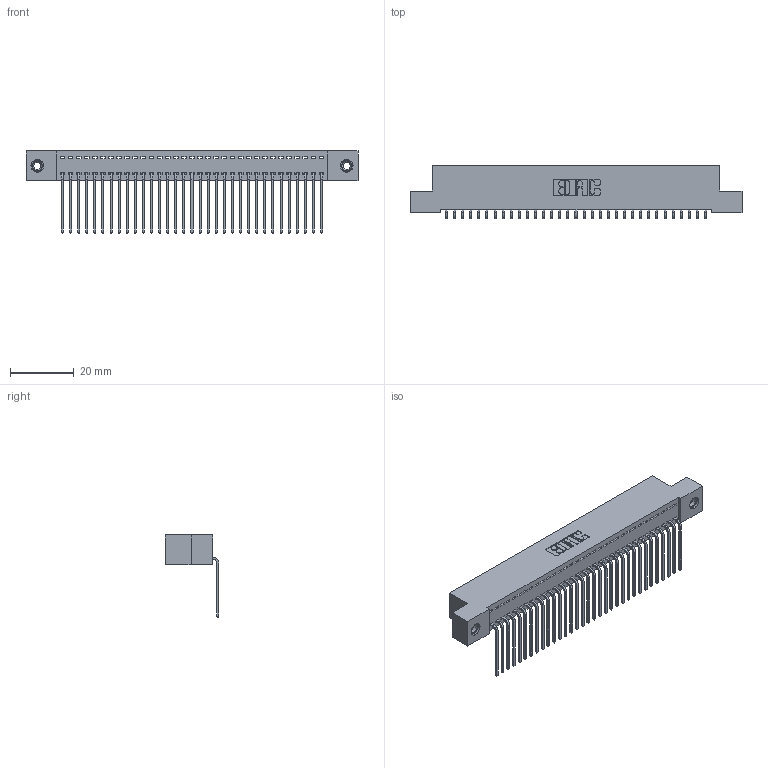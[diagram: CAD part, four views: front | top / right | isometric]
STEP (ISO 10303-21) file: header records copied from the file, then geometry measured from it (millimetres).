
FILE_DESCRIPTION (( 'STEP AP203' ), '1' );
FILE_NAME ('392-033-559-108.STEP', '2018-08-16T01:06:07', ( '' ), ( '' ), 'SwSTEP 2.0', 'SolidWorks 2016', '' );
FILE_SCHEMA (( 'CONFIG_CONTROL_DESIGN' ));
Length unit declared in the file: inch
Products named in the file (4): 342 Part_TI; 345-292-001_558 559 Tail - 1; 345-250-001_345-250-003-102; 392-033-559-108
Assembly tree (36 placements, depth 2):
  392-033-559-108
    342 Part_TI
    345-292-001_558 559 Tail - 1  x33
    345-250-001_345-250-003-102  x2
Bounding box: 104.14 x 16.83 x 25.78 mm (x, y, z)
Volume: 9202.1 mm3; surface area: 13987.1 mm2
Topology: 36 solids, 36 shells, 2150 faces, 6441 edges, 4242 vertices
Faces by surface type: plane 1550, cylinder 584, cone 12, torus 4
Entity records: 22476 total; most frequent: CARTESIAN_POINT 3860, ORIENTED_EDGE 3822, DIRECTION 3307, EDGE_CURVE 1911, LINE 1763, VECTOR 1763, VERTEX_POINT 1268, AXIS2_PLACEMENT_3D 772
